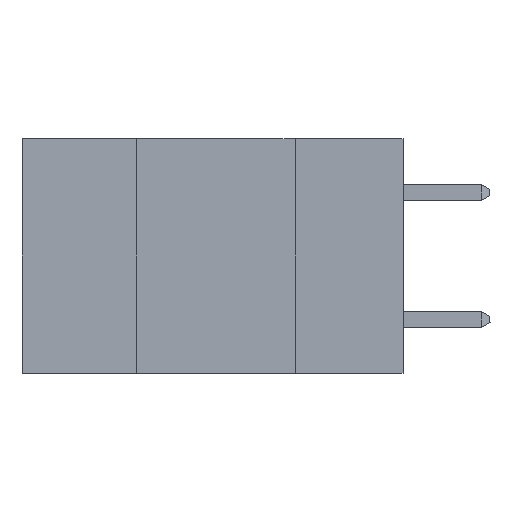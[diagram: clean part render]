
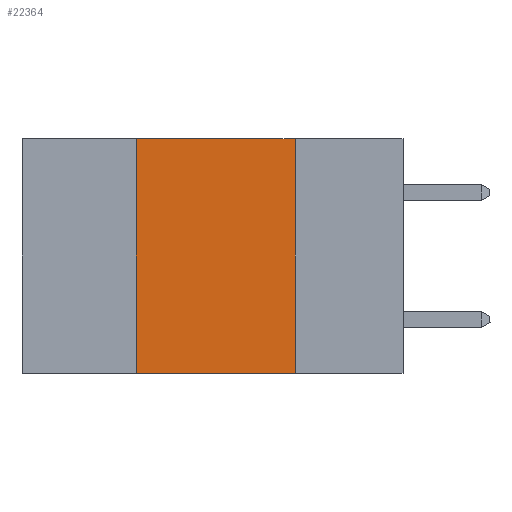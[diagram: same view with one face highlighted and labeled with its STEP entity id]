
A CAD part, left-side view. The second image highlights one B-rep face of the part: STEP entity #22364.
In plain terms, the highlighted planar face has unit normal (-1, 0, 0).
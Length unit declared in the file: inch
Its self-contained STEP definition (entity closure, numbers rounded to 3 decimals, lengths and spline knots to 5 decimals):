
#553 = VECTOR ( 'NONE', #1567, 39.37008 ) ;
#1348 = DIRECTION ( 'NONE',  ( 0., 0., 1. ) ) ;
#1567 = DIRECTION ( 'NONE',  ( 0., -1., 0. ) ) ;
#1632 = CARTESIAN_POINT ( 'NONE',  ( 0., 0.6, 0. ) ) ;
#3824 = VECTOR ( 'NONE', #9288, 39.37008 ) ;
#4134 = VECTOR ( 'NONE', #1348, 39.37008 ) ;
#4606 = CARTESIAN_POINT ( 'NONE',  ( 0., 0.17, 0. ) ) ;
#5395 = LINE ( 'NONE', #1632, #3824 ) ;
#7333 = EDGE_CURVE ( 'NONE', #18010, #16124, #5395, .T. ) ;
#7509 = VERTEX_POINT ( 'NONE', #32082 ) ;
#7785 = DIRECTION ( 'NONE',  ( 0., 0., -1. ) ) ;
#8155 = CARTESIAN_POINT ( 'NONE',  ( 0., 0.42, 0. ) ) ;
#8285 = ORIENTED_EDGE ( 'NONE', *, *, #7333, .F. ) ;
#8925 = EDGE_CURVE ( 'NONE', #7509, #18010, #12113, .T. ) ;
#9288 = DIRECTION ( 'NONE',  ( 0., -1., 0. ) ) ;
#10198 = CARTESIAN_POINT ( 'NONE',  ( 0., 0.17, -0.37 ) ) ;
#11659 = EDGE_CURVE ( 'NONE', #16124, #23668, #24291, .T. ) ;
#11891 = CARTESIAN_POINT ( 'NONE',  ( 0., 0.42, 0. ) ) ;
#12113 = LINE ( 'NONE', #11891, #4134 ) ;
#12254 = PLANE ( 'NONE',  #16647 ) ;
#12749 = ORIENTED_EDGE ( 'NONE', *, *, #14644, .T. ) ;
#12751 = ORIENTED_EDGE ( 'NONE', *, *, #11659, .F. ) ;
#14644 = EDGE_CURVE ( 'NONE', #7509, #23668, #29284, .T. ) ;
#16124 = VERTEX_POINT ( 'NONE', #4606 ) ;
#16647 = AXIS2_PLACEMENT_3D ( 'NONE', #22944, #17775, #30179 ) ;
#17775 = DIRECTION ( 'NONE',  ( 1., 0., 0. ) ) ;
#18010 = VERTEX_POINT ( 'NONE', #8155 ) ;
#18092 = EDGE_LOOP ( 'NONE', ( #12751, #8285, #30626, #12749 ) ) ;
#18408 = CARTESIAN_POINT ( 'NONE',  ( 0., 0.6, -0.37 ) ) ;
#21660 = FACE_OUTER_BOUND ( 'NONE', #18092, .T. ) ;
#22364 = ADVANCED_FACE ( 'NONE', ( #21660 ), #12254, .F. ) ;
#22944 = CARTESIAN_POINT ( 'NONE',  ( 0., 0.6, 0. ) ) ;
#23668 = VERTEX_POINT ( 'NONE', #10198 ) ;
#24291 = LINE ( 'NONE', #25639, #27082 ) ;
#25639 = CARTESIAN_POINT ( 'NONE',  ( 0., 0.17, 0. ) ) ;
#27082 = VECTOR ( 'NONE', #7785, 39.37008 ) ;
#29284 = LINE ( 'NONE', #18408, #553 ) ;
#30179 = DIRECTION ( 'NONE',  ( 0., 0., -1. ) ) ;
#30626 = ORIENTED_EDGE ( 'NONE', *, *, #8925, .F. ) ;
#32082 = CARTESIAN_POINT ( 'NONE',  ( 0., 0.42, -0.37 ) ) ;
